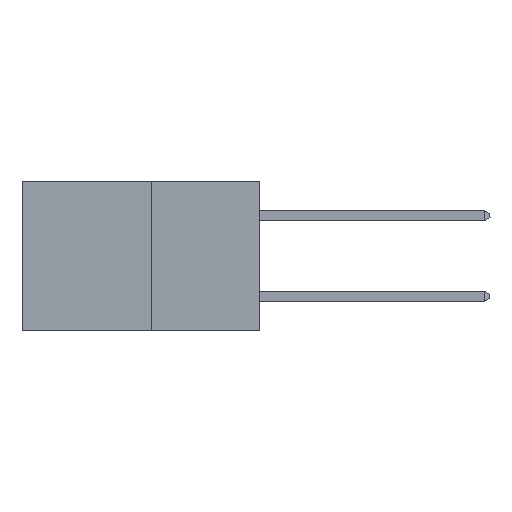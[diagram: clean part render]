
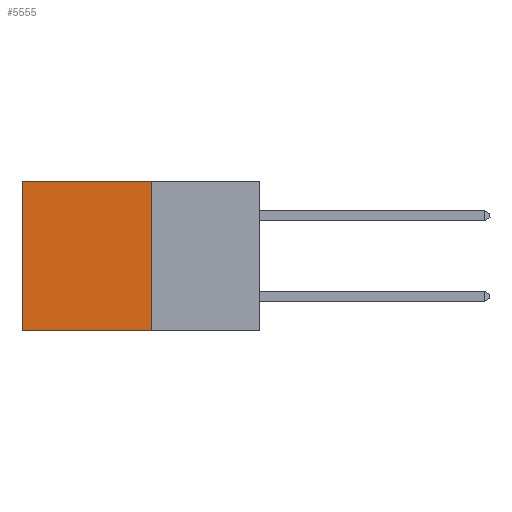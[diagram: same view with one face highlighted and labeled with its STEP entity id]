
A CAD part, left-side view. The second image highlights one B-rep face of the part: STEP entity #5555.
In plain terms, the highlighted planar face has unit normal (-1, 0, 0).
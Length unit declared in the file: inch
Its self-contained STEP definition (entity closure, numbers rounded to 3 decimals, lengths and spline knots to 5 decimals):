
#214 = EDGE_CURVE ( 'NONE', #4744, #382, #3594, .T. ) ;
#249 = ORIENTED_EDGE ( 'NONE', *, *, #3350, .T. ) ;
#251 = ORIENTED_EDGE ( 'NONE', *, *, #324, .F. ) ;
#324 = EDGE_CURVE ( 'NONE', #382, #7409, #4713, .T. ) ;
#336 = CARTESIAN_POINT ( 'NONE',  ( 0.277, 0.27, -0.37 ) ) ;
#382 = VERTEX_POINT ( 'NONE', #5684 ) ;
#472 = VECTOR ( 'NONE', #1100, 39.37008 ) ;
#488 = DIRECTION ( 'NONE',  ( 0., 0., -1. ) ) ;
#666 = DIRECTION ( 'NONE',  ( 0., 1., 0. ) ) ;
#865 = LINE ( 'NONE', #5022, #472 ) ;
#1010 = EDGE_CURVE ( 'NONE', #4744, #5255, #865, .T. ) ;
#1092 = EDGE_LOOP ( 'NONE', ( #249, #251, #2086, #1219 ) ) ;
#1100 = DIRECTION ( 'NONE',  ( 0., 1., 0. ) ) ;
#1219 = ORIENTED_EDGE ( 'NONE', *, *, #1010, .T. ) ;
#1849 = VECTOR ( 'NONE', #488, 39.37008 ) ;
#2070 = DIRECTION ( 'NONE',  ( 0., 0., -1. ) ) ;
#2080 = DIRECTION ( 'NONE',  ( 1., 0., 0. ) ) ;
#2086 = ORIENTED_EDGE ( 'NONE', *, *, #214, .F. ) ;
#2087 = CARTESIAN_POINT ( 'NONE',  ( 0.277, 0.27, -0.37 ) ) ;
#2097 = PLANE ( 'NONE',  #4242 ) ;
#2243 = CARTESIAN_POINT ( 'NONE',  ( 0.277, 0.59, -0.37 ) ) ;
#2784 = VECTOR ( 'NONE', #666, 39.37008 ) ;
#3350 = EDGE_CURVE ( 'NONE', #5255, #7409, #5278, .T. ) ;
#3594 = LINE ( 'NONE', #336, #6692 ) ;
#4242 = AXIS2_PLACEMENT_3D ( 'NONE', #2087, #2080, #2070 ) ;
#4713 = LINE ( 'NONE', #7578, #2784 ) ;
#4744 = VERTEX_POINT ( 'NONE', #4870 ) ;
#4870 = CARTESIAN_POINT ( 'NONE',  ( 0.277, 0.27, 0. ) ) ;
#5022 = CARTESIAN_POINT ( 'NONE',  ( 0.277, 0.27, 0. ) ) ;
#5255 = VERTEX_POINT ( 'NONE', #7021 ) ;
#5278 = LINE ( 'NONE', #5465, #1849 ) ;
#5334 = FACE_OUTER_BOUND ( 'NONE', #1092, .T. ) ;
#5465 = CARTESIAN_POINT ( 'NONE',  ( 0.277, 0.59, -0.37 ) ) ;
#5555 = ADVANCED_FACE ( 'NONE', ( #5334 ), #2097, .F. ) ;
#5684 = CARTESIAN_POINT ( 'NONE',  ( 0.277, 0.27, -0.37 ) ) ;
#5882 = DIRECTION ( 'NONE',  ( 0., 0., -1. ) ) ;
#6692 = VECTOR ( 'NONE', #5882, 39.37008 ) ;
#7021 = CARTESIAN_POINT ( 'NONE',  ( 0.277, 0.59, 0. ) ) ;
#7409 = VERTEX_POINT ( 'NONE', #2243 ) ;
#7578 = CARTESIAN_POINT ( 'NONE',  ( 0.277, 0.27, -0.37 ) ) ;
